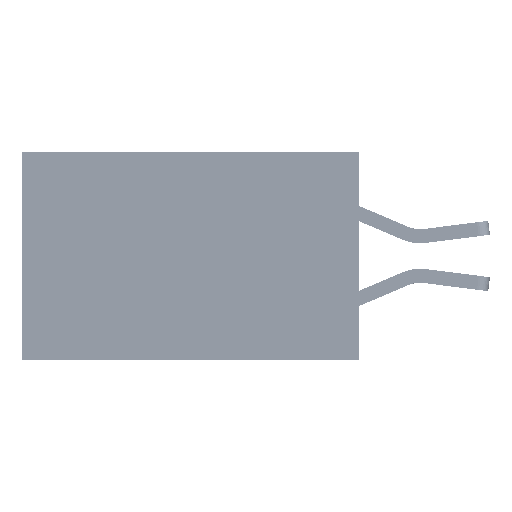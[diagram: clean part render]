
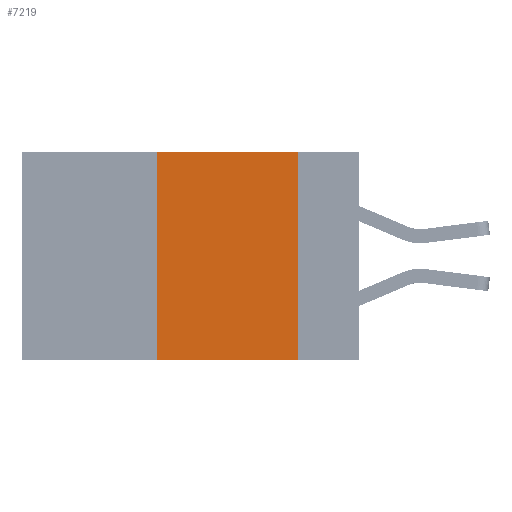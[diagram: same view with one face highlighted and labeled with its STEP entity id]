
A CAD part, left-side view. The second image highlights one B-rep face of the part: STEP entity #7219.
In plain terms, the highlighted planar face has unit normal (-1, 0, 0).
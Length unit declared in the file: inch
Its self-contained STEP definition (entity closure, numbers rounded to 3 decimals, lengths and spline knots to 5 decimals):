
#211 = PLANE ( 'NONE',  #33246 ) ;
#502 = DIRECTION ( 'NONE',  ( 0., -1., 0. ) ) ;
#1364 = LINE ( 'NONE', #16341, #9876 ) ;
#4857 = CARTESIAN_POINT ( 'NONE',  ( 0., 0.36, 0. ) ) ;
#5617 = VECTOR ( 'NONE', #14051, 39.37008 ) ;
#7219 = ADVANCED_FACE ( 'NONE', ( #24707 ), #211, .F. ) ;
#7839 = LINE ( 'NONE', #28223, #19743 ) ;
#8834 = VERTEX_POINT ( 'NONE', #17939 ) ;
#8991 = EDGE_CURVE ( 'NONE', #18215, #36002, #1364, .T. ) ;
#9876 = VECTOR ( 'NONE', #10105, 39.37008 ) ;
#10105 = DIRECTION ( 'NONE',  ( 0., -1., 0. ) ) ;
#10549 = DIRECTION ( 'NONE',  ( 0., 0., -1. ) ) ;
#13717 = LINE ( 'NONE', #20138, #5617 ) ;
#14051 = DIRECTION ( 'NONE',  ( 0., 0., -1. ) ) ;
#16274 = EDGE_CURVE ( 'NONE', #18215, #24808, #36114, .T. ) ;
#16341 = CARTESIAN_POINT ( 'NONE',  ( 0., 0.6, -0.37 ) ) ;
#17405 = EDGE_CURVE ( 'NONE', #8834, #36002, #13717, .T. ) ;
#17939 = CARTESIAN_POINT ( 'NONE',  ( 0., 0.11, 0. ) ) ;
#18215 = VERTEX_POINT ( 'NONE', #23158 ) ;
#18789 = CARTESIAN_POINT ( 'NONE',  ( 0., 0.36, 0. ) ) ;
#19253 = ORIENTED_EDGE ( 'NONE', *, *, #32103, .F. ) ;
#19612 = DIRECTION ( 'NONE',  ( 0., 0., 1. ) ) ;
#19743 = VECTOR ( 'NONE', #502, 39.37008 ) ;
#19914 = CARTESIAN_POINT ( 'NONE',  ( 0., 0.11, -0.37 ) ) ;
#20138 = CARTESIAN_POINT ( 'NONE',  ( 0., 0.11, 0. ) ) ;
#20720 = ORIENTED_EDGE ( 'NONE', *, *, #8991, .T. ) ;
#23158 = CARTESIAN_POINT ( 'NONE',  ( 0., 0.36, -0.37 ) ) ;
#23874 = DIRECTION ( 'NONE',  ( 1., 0., 0. ) ) ;
#24707 = FACE_OUTER_BOUND ( 'NONE', #34462, .T. ) ;
#24808 = VERTEX_POINT ( 'NONE', #18789 ) ;
#25567 = CARTESIAN_POINT ( 'NONE',  ( 0., 0.6, 0. ) ) ;
#28031 = VECTOR ( 'NONE', #19612, 39.37008 ) ;
#28223 = CARTESIAN_POINT ( 'NONE',  ( 0., 0.6, 0. ) ) ;
#28732 = ORIENTED_EDGE ( 'NONE', *, *, #16274, .F. ) ;
#32103 = EDGE_CURVE ( 'NONE', #24808, #8834, #7839, .T. ) ;
#33246 = AXIS2_PLACEMENT_3D ( 'NONE', #25567, #23874, #10549 ) ;
#34462 = EDGE_LOOP ( 'NONE', ( #35593, #19253, #28732, #20720 ) ) ;
#35593 = ORIENTED_EDGE ( 'NONE', *, *, #17405, .F. ) ;
#36002 = VERTEX_POINT ( 'NONE', #19914 ) ;
#36114 = LINE ( 'NONE', #4857, #28031 ) ;
